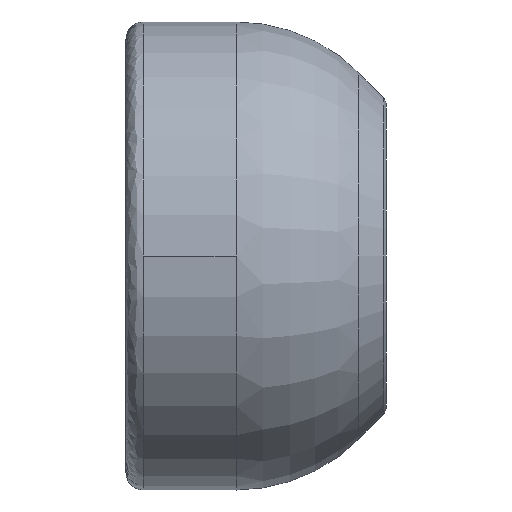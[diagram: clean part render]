
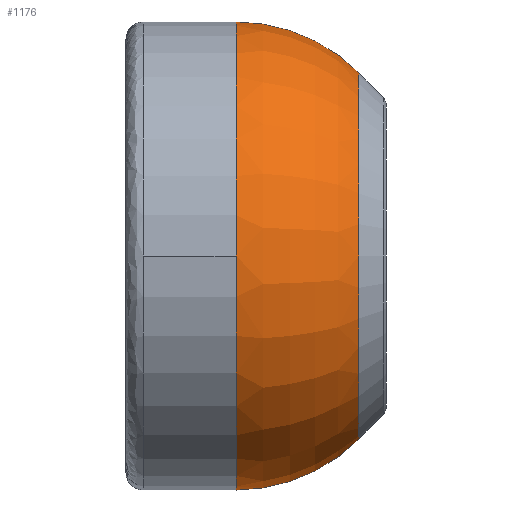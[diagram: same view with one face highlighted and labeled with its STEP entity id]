
A CAD part, front view. The second image highlights one B-rep face of the part: STEP entity #1176.
In plain terms, the highlighted toroidal (fillet/blend) face has major radius 3.5 mm and minor radius 10 mm.
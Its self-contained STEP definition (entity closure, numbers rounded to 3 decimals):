
#112 = DIRECTION ( 'NONE',  ( 0., 0., 1. ) ) ;
#158 = CIRCLE ( 'NONE', #1075, 10.571 ) ;
#170 = CARTESIAN_POINT ( 'NONE',  ( -160.453, 46.521, 11.571 ) ) ;
#175 = EDGE_CURVE ( 'NONE', #1241, #820, #978, .T. ) ;
#185 = CIRCLE ( 'NONE', #620, 13.5 ) ;
#266 = EDGE_CURVE ( 'NONE', #1241, #779, #158, .T. ) ;
#301 = EDGE_CURVE ( 'NONE', #563, #611, #185, .T. ) ;
#323 = EDGE_CURVE ( 'NONE', #779, #563, #1052, .T. ) ;
#403 = AXIS2_PLACEMENT_3D ( 'NONE', #529, #624, #1143 ) ;
#443 = ORIENTED_EDGE ( 'NONE', *, *, #323, .F. ) ;
#446 = DIRECTION ( 'NONE',  ( 0., 1., 0. ) ) ;
#461 = DIRECTION ( 'NONE',  ( 0., 0., -1. ) ) ;
#480 = CARTESIAN_POINT ( 'NONE',  ( -167.524, 46.521, 1. ) ) ;
#528 = CIRCLE ( 'NONE', #403, 13.5 ) ;
#529 = CARTESIAN_POINT ( 'NONE',  ( -167.524, 46.521, 1. ) ) ;
#554 = AXIS2_PLACEMENT_3D ( 'NONE', #480, #1235, #112 ) ;
#563 = VERTEX_POINT ( 'NONE', #729 ) ;
#569 = CARTESIAN_POINT ( 'NONE',  ( -167.524, 46.521, -2.5 ) ) ;
#611 = VERTEX_POINT ( 'NONE', #1184 ) ;
#620 = AXIS2_PLACEMENT_3D ( 'NONE', #835, #1196, #1218 ) ;
#624 = DIRECTION ( 'NONE',  ( -1., 0., 0. ) ) ;
#655 = CARTESIAN_POINT ( 'NONE',  ( -167.524, 46.521, 14.5 ) ) ;
#705 = DIRECTION ( 'NONE',  ( 0., 0., -1. ) ) ;
#713 = CARTESIAN_POINT ( 'NONE',  ( -160.453, 46.521, 1. ) ) ;
#729 = CARTESIAN_POINT ( 'NONE',  ( -167.524, 46.521, -12.5 ) ) ;
#779 = VERTEX_POINT ( 'NONE', #1258 ) ;
#811 = EDGE_LOOP ( 'NONE', ( #443, #1063, #1134, #1570, #1183 ) ) ;
#820 = VERTEX_POINT ( 'NONE', #655 ) ;
#835 = CARTESIAN_POINT ( 'NONE',  ( -167.524, 46.521, 1. ) ) ;
#922 = AXIS2_PLACEMENT_3D ( 'NONE', #966, #1458, #705 ) ;
#966 = CARTESIAN_POINT ( 'NONE',  ( -167.524, 46.521, 4.5 ) ) ;
#978 = CIRCLE ( 'NONE', #922, 10. ) ;
#998 = FACE_OUTER_BOUND ( 'NONE', #811, .T. ) ;
#1052 = CIRCLE ( 'NONE', #1536, 10. ) ;
#1063 = ORIENTED_EDGE ( 'NONE', *, *, #266, .F. ) ;
#1075 = AXIS2_PLACEMENT_3D ( 'NONE', #713, #1316, #461 ) ;
#1134 = ORIENTED_EDGE ( 'NONE', *, *, #175, .T. ) ;
#1143 = DIRECTION ( 'NONE',  ( 0., 0., -1. ) ) ;
#1176 = ADVANCED_FACE ( 'NONE', ( #998 ), #1255, .T. ) ;
#1183 = ORIENTED_EDGE ( 'NONE', *, *, #301, .F. ) ;
#1184 = CARTESIAN_POINT ( 'NONE',  ( -167.524, 33.021, 1. ) ) ;
#1196 = DIRECTION ( 'NONE',  ( -1., 0., 0. ) ) ;
#1203 = DIRECTION ( 'NONE',  ( 0., 0., 1. ) ) ;
#1218 = DIRECTION ( 'NONE',  ( 0., 0., -1. ) ) ;
#1235 = DIRECTION ( 'NONE',  ( -1., 0., 0. ) ) ;
#1241 = VERTEX_POINT ( 'NONE', #170 ) ;
#1255 = TOROIDAL_SURFACE ( 'NONE', #554, 3.5, 10. ) ;
#1258 = CARTESIAN_POINT ( 'NONE',  ( -160.453, 46.521, -9.571 ) ) ;
#1316 = DIRECTION ( 'NONE',  ( 1., 0., 0. ) ) ;
#1458 = DIRECTION ( 'NONE',  ( 0., -1., 0. ) ) ;
#1507 = EDGE_CURVE ( 'NONE', #611, #820, #528, .T. ) ;
#1536 = AXIS2_PLACEMENT_3D ( 'NONE', #569, #446, #1203 ) ;
#1570 = ORIENTED_EDGE ( 'NONE', *, *, #1507, .F. ) ;
